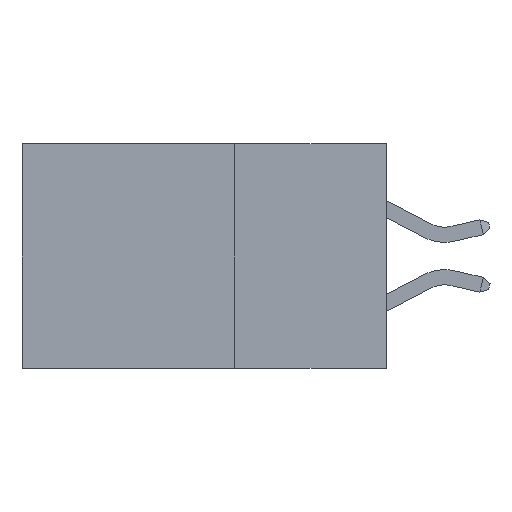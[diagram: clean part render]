
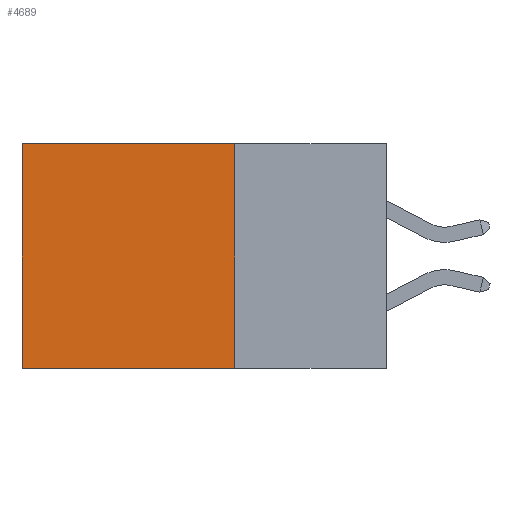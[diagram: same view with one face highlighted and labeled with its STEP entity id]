
A CAD part, left-side view. The second image highlights one B-rep face of the part: STEP entity #4689.
In plain terms, the highlighted planar face has unit normal (-1, 0, 0).
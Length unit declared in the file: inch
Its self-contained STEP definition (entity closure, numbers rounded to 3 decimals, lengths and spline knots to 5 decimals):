
#9 = CARTESIAN_POINT ( 'NONE',  ( 0.2615, 0.6, 0. ) ) ;
#108 = DIRECTION ( 'NONE',  ( 0., 0., -1. ) ) ;
#1156 = CARTESIAN_POINT ( 'NONE',  ( 0.2615, 0.25, -0.37 ) ) ;
#2307 = EDGE_CURVE ( 'NONE', #15219, #17611, #22568, .T. ) ;
#2871 = CARTESIAN_POINT ( 'NONE',  ( 0.2615, 0.25, -0.37 ) ) ;
#3107 = EDGE_LOOP ( 'NONE', ( #20990, #21774, #18564, #17866 ) ) ;
#4689 = ADVANCED_FACE ( 'NONE', ( #15852 ), #19244, .F. ) ;
#6237 = CARTESIAN_POINT ( 'NONE',  ( 0.2615, 0.25, -0.37 ) ) ;
#6940 = VECTOR ( 'NONE', #11121, 39.37008 ) ;
#7747 = CARTESIAN_POINT ( 'NONE',  ( 0.2615, 0.25, 0. ) ) ;
#8049 = LINE ( 'NONE', #13122, #19082 ) ;
#8139 = DIRECTION ( 'NONE',  ( 1., 0., 0. ) ) ;
#8250 = CARTESIAN_POINT ( 'NONE',  ( 0.2615, 0.6, -0.37 ) ) ;
#9232 = CARTESIAN_POINT ( 'NONE',  ( 0.2615, 0.25, -0.37 ) ) ;
#9525 = VERTEX_POINT ( 'NONE', #7747 ) ;
#11121 = DIRECTION ( 'NONE',  ( 0., 1., 0. ) ) ;
#12073 = EDGE_CURVE ( 'NONE', #12906, #17611, #21726, .T. ) ;
#12794 = VECTOR ( 'NONE', #108, 39.37008 ) ;
#12906 = VERTEX_POINT ( 'NONE', #2871 ) ;
#13122 = CARTESIAN_POINT ( 'NONE',  ( 0.2615, 0.25, 0. ) ) ;
#13265 = VECTOR ( 'NONE', #16311, 39.37008 ) ;
#14276 = CARTESIAN_POINT ( 'NONE',  ( 0.2615, 0.6, -0.37 ) ) ;
#15219 = VERTEX_POINT ( 'NONE', #9 ) ;
#15650 = EDGE_CURVE ( 'NONE', #9525, #12906, #23604, .T. ) ;
#15852 = FACE_OUTER_BOUND ( 'NONE', #3107, .T. ) ;
#16311 = DIRECTION ( 'NONE',  ( 0., 0., -1. ) ) ;
#17611 = VERTEX_POINT ( 'NONE', #8250 ) ;
#17866 = ORIENTED_EDGE ( 'NONE', *, *, #18643, .T. ) ;
#18427 = AXIS2_PLACEMENT_3D ( 'NONE', #6237, #8139, #21082 ) ;
#18564 = ORIENTED_EDGE ( 'NONE', *, *, #15650, .F. ) ;
#18643 = EDGE_CURVE ( 'NONE', #9525, #15219, #8049, .T. ) ;
#19082 = VECTOR ( 'NONE', #24082, 39.37008 ) ;
#19244 = PLANE ( 'NONE',  #18427 ) ;
#20990 = ORIENTED_EDGE ( 'NONE', *, *, #2307, .T. ) ;
#21082 = DIRECTION ( 'NONE',  ( 0., 0., -1. ) ) ;
#21726 = LINE ( 'NONE', #9232, #6940 ) ;
#21774 = ORIENTED_EDGE ( 'NONE', *, *, #12073, .F. ) ;
#22568 = LINE ( 'NONE', #14276, #12794 ) ;
#23604 = LINE ( 'NONE', #1156, #13265 ) ;
#24082 = DIRECTION ( 'NONE',  ( 0., 1., 0. ) ) ;
